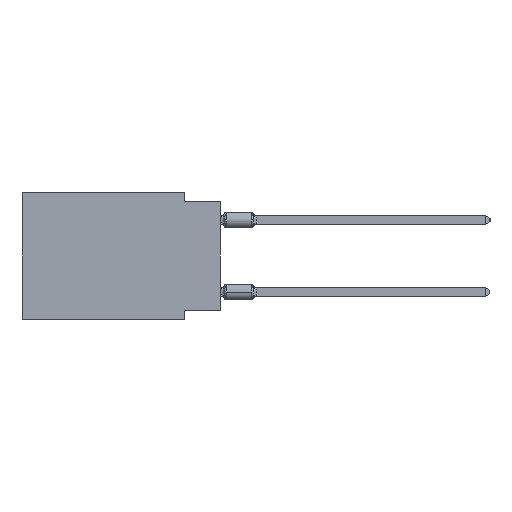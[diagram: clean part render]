
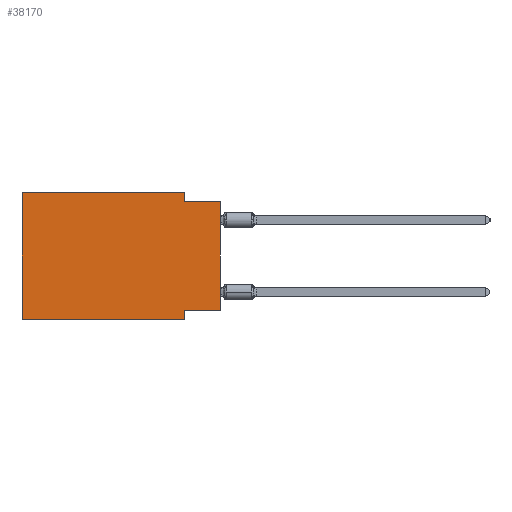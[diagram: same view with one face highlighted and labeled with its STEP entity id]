
A CAD part, left-side view. The second image highlights one B-rep face of the part: STEP entity #38170.
In plain terms, the highlighted planar face has unit normal (-1, 0, 0).
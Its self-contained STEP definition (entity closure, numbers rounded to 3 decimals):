
#551 = VECTOR ( 'NONE', #19076, 1000. ) ;
#965 = CARTESIAN_POINT ( 'NONE',  ( 0., 2.54, -8.89 ) ) ;
#1668 = CARTESIAN_POINT ( 'NONE',  ( 0., 13.97, 0. ) ) ;
#1985 = CARTESIAN_POINT ( 'NONE',  ( 0., 0., -0.635 ) ) ;
#3250 = ORIENTED_EDGE ( 'NONE', *, *, #20170, .F. ) ;
#3953 = EDGE_CURVE ( 'NONE', #41520, #36975, #12650, .T. ) ;
#5380 = DIRECTION ( 'NONE',  ( 0., 0., 1. ) ) ;
#5843 = DIRECTION ( 'NONE',  ( 1., 0., 0. ) ) ;
#5925 = CARTESIAN_POINT ( 'NONE',  ( 0., 2.54, -8.255 ) ) ;
#7236 = AXIS2_PLACEMENT_3D ( 'NONE', #24054, #5843, #30657 ) ;
#8070 = LINE ( 'NONE', #30052, #28150 ) ;
#8408 = DIRECTION ( 'NONE',  ( 0., 0., 1. ) ) ;
#8548 = DIRECTION ( 'NONE',  ( 0., 0., -1. ) ) ;
#10634 = LINE ( 'NONE', #35473, #13194 ) ;
#11996 = CARTESIAN_POINT ( 'NONE',  ( 0., 13.97, -8.89 ) ) ;
#12650 = LINE ( 'NONE', #27064, #38387 ) ;
#13194 = VECTOR ( 'NONE', #14626, 1000. ) ;
#14626 = DIRECTION ( 'NONE',  ( 0., 1., 0. ) ) ;
#14766 = VERTEX_POINT ( 'NONE', #1668 ) ;
#14817 = VERTEX_POINT ( 'NONE', #5925 ) ;
#14904 = LINE ( 'NONE', #965, #15310 ) ;
#14971 = EDGE_CURVE ( 'NONE', #41520, #14817, #10634, .T. ) ;
#14995 = CARTESIAN_POINT ( 'NONE',  ( 0., 0., -8.255 ) ) ;
#15029 = LINE ( 'NONE', #29681, #36825 ) ;
#15310 = VECTOR ( 'NONE', #8548, 1000. ) ;
#16242 = ORIENTED_EDGE ( 'NONE', *, *, #35979, .F. ) ;
#16430 = VERTEX_POINT ( 'NONE', #38514 ) ;
#16784 = ORIENTED_EDGE ( 'NONE', *, *, #27288, .F. ) ;
#19076 = DIRECTION ( 'NONE',  ( 0., -1., 0. ) ) ;
#20170 = EDGE_CURVE ( 'NONE', #30694, #36975, #8070, .T. ) ;
#20268 = LINE ( 'NONE', #34449, #21527 ) ;
#20500 = ORIENTED_EDGE ( 'NONE', *, *, #45595, .F. ) ;
#20656 = CARTESIAN_POINT ( 'NONE',  ( 0., 2.54, -0.635 ) ) ;
#20672 = VECTOR ( 'NONE', #22752, 1000. ) ;
#21527 = VECTOR ( 'NONE', #5380, 1000. ) ;
#22280 = CARTESIAN_POINT ( 'NONE',  ( 0., 13.97, 0. ) ) ;
#22752 = DIRECTION ( 'NONE',  ( 0., -1., 0. ) ) ;
#24054 = CARTESIAN_POINT ( 'NONE',  ( 0., 13.97, 0. ) ) ;
#25407 = ORIENTED_EDGE ( 'NONE', *, *, #14971, .F. ) ;
#25480 = ORIENTED_EDGE ( 'NONE', *, *, #31220, .F. ) ;
#26011 = VERTEX_POINT ( 'NONE', #34365 ) ;
#26264 = VERTEX_POINT ( 'NONE', #40714 ) ;
#26872 = LINE ( 'NONE', #11996, #551 ) ;
#27064 = CARTESIAN_POINT ( 'NONE',  ( 0., 0., 0. ) ) ;
#27288 = EDGE_CURVE ( 'NONE', #14817, #16430, #14904, .T. ) ;
#27879 = ORIENTED_EDGE ( 'NONE', *, *, #39762, .T. ) ;
#28150 = VECTOR ( 'NONE', #37645, 1000. ) ;
#29681 = CARTESIAN_POINT ( 'NONE',  ( 0., 2.54, 0. ) ) ;
#29821 = LINE ( 'NONE', #22280, #20672 ) ;
#30052 = CARTESIAN_POINT ( 'NONE',  ( 0., 0., -0.635 ) ) ;
#30657 = DIRECTION ( 'NONE',  ( 0., 0., -1. ) ) ;
#30694 = VERTEX_POINT ( 'NONE', #20656 ) ;
#31220 = EDGE_CURVE ( 'NONE', #26264, #30694, #15029, .T. ) ;
#32986 = EDGE_LOOP ( 'NONE', ( #39560, #3250, #25480, #20500, #16242, #27879, #16784, #25407 ) ) ;
#34365 = CARTESIAN_POINT ( 'NONE',  ( 0., 13.97, -8.89 ) ) ;
#34449 = CARTESIAN_POINT ( 'NONE',  ( 0., 13.97, 0. ) ) ;
#35473 = CARTESIAN_POINT ( 'NONE',  ( 0., 0., -8.255 ) ) ;
#35979 = EDGE_CURVE ( 'NONE', #26011, #14766, #20268, .T. ) ;
#36332 = DIRECTION ( 'NONE',  ( 0., 0., -1. ) ) ;
#36825 = VECTOR ( 'NONE', #36332, 1000. ) ;
#36975 = VERTEX_POINT ( 'NONE', #1985 ) ;
#37645 = DIRECTION ( 'NONE',  ( 0., -1., 0. ) ) ;
#38170 = ADVANCED_FACE ( 'NONE', ( #38245 ), #41099, .F. ) ;
#38245 = FACE_OUTER_BOUND ( 'NONE', #32986, .T. ) ;
#38387 = VECTOR ( 'NONE', #8408, 1000. ) ;
#38514 = CARTESIAN_POINT ( 'NONE',  ( 0., 2.54, -8.89 ) ) ;
#39560 = ORIENTED_EDGE ( 'NONE', *, *, #3953, .T. ) ;
#39762 = EDGE_CURVE ( 'NONE', #26011, #16430, #26872, .T. ) ;
#40714 = CARTESIAN_POINT ( 'NONE',  ( 0., 2.54, 0. ) ) ;
#41099 = PLANE ( 'NONE',  #7236 ) ;
#41520 = VERTEX_POINT ( 'NONE', #14995 ) ;
#45595 = EDGE_CURVE ( 'NONE', #14766, #26264, #29821, .T. ) ;
